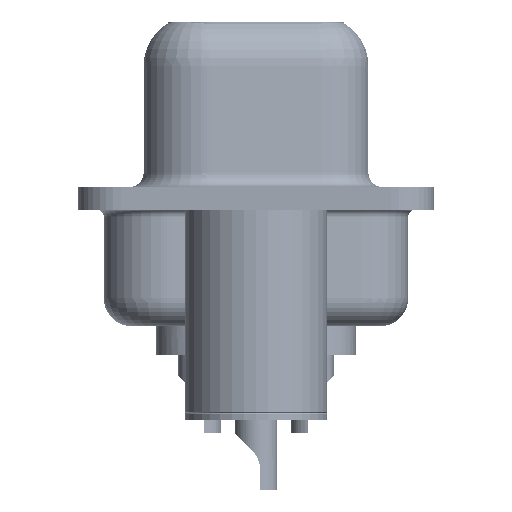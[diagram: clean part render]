
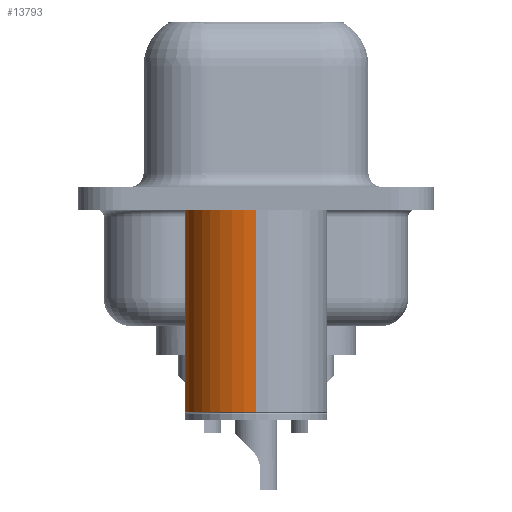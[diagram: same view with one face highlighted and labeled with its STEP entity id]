
A CAD part, left-side view. The second image highlights one B-rep face of the part: STEP entity #13793.
In plain terms, the highlighted cylindrical face has radius 2.5 mm (diameter 5 mm), a partial arc.
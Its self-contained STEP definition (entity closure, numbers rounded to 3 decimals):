
#31 = ORIENTED_EDGE ( 'NONE', *, *, #14079, .T. ) ;
#5060 = EDGE_CURVE ( 'NONE', #16076, #25239, #6636, .T. ) ;
#5401 = AXIS2_PLACEMENT_3D ( 'NONE', #12449, #30427, #12840 ) ;
#5653 = DIRECTION ( 'NONE',  ( 0., 0., 1. ) ) ;
#6041 = CIRCLE ( 'NONE', #5401, 2.5 ) ;
#6636 = LINE ( 'NONE', #20892, #20171 ) ;
#12287 = ORIENTED_EDGE ( 'NONE', *, *, #5060, .F. ) ;
#12310 = EDGE_LOOP ( 'NONE', ( #16362, #31, #32888, #12287 ) ) ;
#12449 = CARTESIAN_POINT ( 'NONE',  ( 0., 0., -7.525 ) ) ;
#12840 = DIRECTION ( 'NONE',  ( 1., 0., 0. ) ) ;
#13793 = ADVANCED_FACE ( 'NONE', ( #20872 ), #23231, .T. ) ;
#14079 = EDGE_CURVE ( 'NONE', #17031, #33269, #24764, .T. ) ;
#14812 = CARTESIAN_POINT ( 'NONE',  ( 2.5, 0., -7.525 ) ) ;
#14891 = CARTESIAN_POINT ( 'NONE',  ( -2.5, 0., -0.4 ) ) ;
#16076 = VERTEX_POINT ( 'NONE', #14812 ) ;
#16362 = ORIENTED_EDGE ( 'NONE', *, *, #17695, .T. ) ;
#17031 = VERTEX_POINT ( 'NONE', #38313 ) ;
#17695 = EDGE_CURVE ( 'NONE', #16076, #17031, #6041, .T. ) ;
#19887 = CARTESIAN_POINT ( 'NONE',  ( -2.5, 0., 0.581 ) ) ;
#20171 = VECTOR ( 'NONE', #24017, 1000. ) ;
#20872 = FACE_OUTER_BOUND ( 'NONE', #12310, .T. ) ;
#20892 = CARTESIAN_POINT ( 'NONE',  ( 2.5, 0., 0.581 ) ) ;
#22998 = DIRECTION ( 'NONE',  ( 0., 0., 1. ) ) ;
#23231 = CYLINDRICAL_SURFACE ( 'NONE', #28945, 2.5 ) ;
#23937 = VECTOR ( 'NONE', #22998, 1000. ) ;
#24017 = DIRECTION ( 'NONE',  ( 0., 0., 1. ) ) ;
#24062 = EDGE_CURVE ( 'NONE', #25239, #33269, #28181, .T. ) ;
#24083 = CARTESIAN_POINT ( 'NONE',  ( 0., 0., -0.4 ) ) ;
#24764 = LINE ( 'NONE', #19887, #23937 ) ;
#25239 = VERTEX_POINT ( 'NONE', #25533 ) ;
#25533 = CARTESIAN_POINT ( 'NONE',  ( 2.5, 0., -0.4 ) ) ;
#28181 = CIRCLE ( 'NONE', #30037, 2.5 ) ;
#28945 = AXIS2_PLACEMENT_3D ( 'NONE', #38286, #5653, #29472 ) ;
#29472 = DIRECTION ( 'NONE',  ( 1., 0., 0. ) ) ;
#30037 = AXIS2_PLACEMENT_3D ( 'NONE', #24083, #36018, #30141 ) ;
#30141 = DIRECTION ( 'NONE',  ( 1., 0., 0. ) ) ;
#30427 = DIRECTION ( 'NONE',  ( 0., 0., 1. ) ) ;
#32888 = ORIENTED_EDGE ( 'NONE', *, *, #24062, .F. ) ;
#33269 = VERTEX_POINT ( 'NONE', #14891 ) ;
#36018 = DIRECTION ( 'NONE',  ( 0., 0., 1. ) ) ;
#38286 = CARTESIAN_POINT ( 'NONE',  ( 0., 0., 0.581 ) ) ;
#38313 = CARTESIAN_POINT ( 'NONE',  ( -2.5, 0., -7.525 ) ) ;
